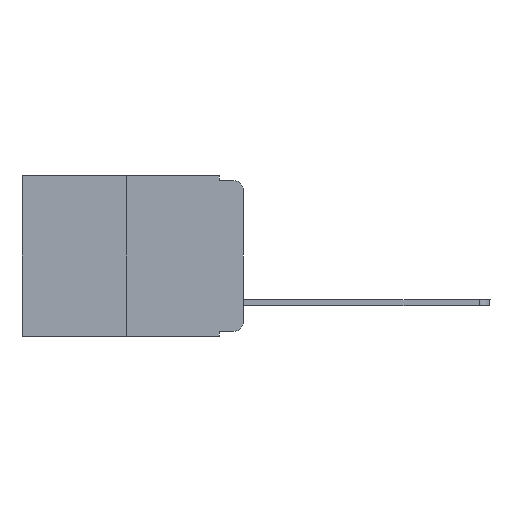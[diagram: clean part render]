
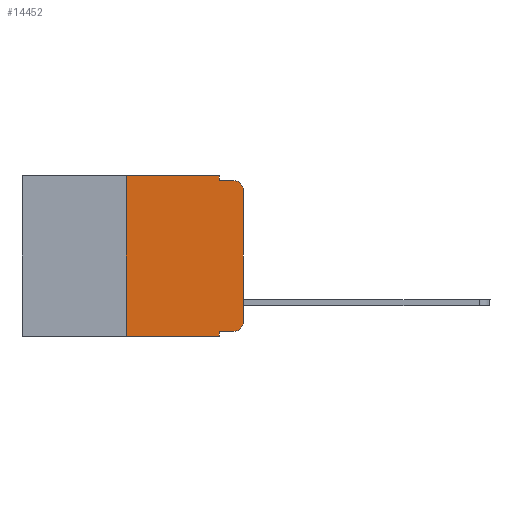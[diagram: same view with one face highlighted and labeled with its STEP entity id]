
A CAD part, left-side view. The second image highlights one B-rep face of the part: STEP entity #14452.
In plain terms, the highlighted planar face has unit normal (-1, 0, 0).
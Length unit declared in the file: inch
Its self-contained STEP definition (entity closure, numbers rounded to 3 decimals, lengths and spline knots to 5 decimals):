
#571 = DIRECTION ( 'NONE',  ( 1., 0., 0. ) ) ;
#807 = VECTOR ( 'NONE', #3811, 39.37008 ) ;
#868 = ORIENTED_EDGE ( 'NONE', *, *, #10553, .T. ) ;
#1630 = EDGE_CURVE ( 'NONE', #2221, #11565, #3370, .T. ) ;
#1830 = CARTESIAN_POINT ( 'NONE',  ( 0., 0.473, 0. ) ) ;
#1958 = VECTOR ( 'NONE', #14750, 39.37008 ) ;
#2143 = PLANE ( 'NONE',  #5240 ) ;
#2221 = VERTEX_POINT ( 'NONE', #19206 ) ;
#2277 = CARTESIAN_POINT ( 'NONE',  ( 0., 0.051, -0.01 ) ) ;
#2434 = DIRECTION ( 'NONE',  ( 0., 0., -1. ) ) ;
#2792 = CARTESIAN_POINT ( 'NONE',  ( 0., 0.051, 0. ) ) ;
#2805 = VECTOR ( 'NONE', #14212, 39.37008 ) ;
#3166 = ORIENTED_EDGE ( 'NONE', *, *, #14502, .T. ) ;
#3370 = LINE ( 'NONE', #14201, #13735 ) ;
#3387 = VECTOR ( 'NONE', #5012, 39.37008 ) ;
#3401 = ORIENTED_EDGE ( 'NONE', *, *, #6089, .T. ) ;
#3436 = VERTEX_POINT ( 'NONE', #17868 ) ;
#3811 = DIRECTION ( 'NONE',  ( 0., -1., 0. ) ) ;
#4032 = LINE ( 'NONE', #1830, #6422 ) ;
#4248 = VERTEX_POINT ( 'NONE', #9648 ) ;
#4620 = VERTEX_POINT ( 'NONE', #11675 ) ;
#4921 = DIRECTION ( 'NONE',  ( 0., 0., 1. ) ) ;
#4950 = CARTESIAN_POINT ( 'NONE',  ( 0., 0.051, -0.343 ) ) ;
#5012 = DIRECTION ( 'NONE',  ( 0., -1., 0. ) ) ;
#5240 = AXIS2_PLACEMENT_3D ( 'NONE', #8316, #571, #12733 ) ;
#5625 = CARTESIAN_POINT ( 'NONE',  ( 0., 0., -0.03 ) ) ;
#6017 = LINE ( 'NONE', #12863, #3387 ) ;
#6089 = EDGE_CURVE ( 'NONE', #4248, #16490, #9199, .T. ) ;
#6422 = VECTOR ( 'NONE', #15561, 39.37008 ) ;
#6891 = ORIENTED_EDGE ( 'NONE', *, *, #16332, .T. ) ;
#8015 = CARTESIAN_POINT ( 'NONE',  ( 0., 0., 0. ) ) ;
#8316 = CARTESIAN_POINT ( 'NONE',  ( 0., 0.473, 0. ) ) ;
#8331 = LINE ( 'NONE', #19037, #2805 ) ;
#8610 = DIRECTION ( 'NONE',  ( -1., 0., 0. ) ) ;
#9040 = CARTESIAN_POINT ( 'NONE',  ( 0., 0.02, -0.01 ) ) ;
#9199 = LINE ( 'NONE', #8015, #15433 ) ;
#9222 = VERTEX_POINT ( 'NONE', #9040 ) ;
#9281 = ORIENTED_EDGE ( 'NONE', *, *, #16196, .F. ) ;
#9462 = ORIENTED_EDGE ( 'NONE', *, *, #19541, .F. ) ;
#9648 = CARTESIAN_POINT ( 'NONE',  ( 0., 0., -0.313 ) ) ;
#9707 = EDGE_CURVE ( 'NONE', #16307, #17786, #10130, .T. ) ;
#9800 = CARTESIAN_POINT ( 'NONE',  ( 0., 0.051, 0. ) ) ;
#9999 = CARTESIAN_POINT ( 'NONE',  ( 0., 0.051, -0.333 ) ) ;
#10130 = LINE ( 'NONE', #2792, #1958 ) ;
#10535 = ORIENTED_EDGE ( 'NONE', *, *, #11070, .T. ) ;
#10553 = EDGE_CURVE ( 'NONE', #16490, #9222, #12452, .T. ) ;
#11070 = EDGE_CURVE ( 'NONE', #4620, #4248, #13889, .T. ) ;
#11306 = FACE_OUTER_BOUND ( 'NONE', #15638, .T. ) ;
#11326 = ORIENTED_EDGE ( 'NONE', *, *, #9707, .F. ) ;
#11565 = VERTEX_POINT ( 'NONE', #14657 ) ;
#11675 = CARTESIAN_POINT ( 'NONE',  ( 0., 0.02, -0.333 ) ) ;
#11723 = CARTESIAN_POINT ( 'NONE',  ( 0., 0.02, -0.03 ) ) ;
#11850 = DIRECTION ( 'NONE',  ( 0., 0., -1. ) ) ;
#12158 = VERTEX_POINT ( 'NONE', #4950 ) ;
#12452 = CIRCLE ( 'NONE', #16785, 0.02 ) ;
#12646 = LINE ( 'NONE', #9999, #14107 ) ;
#12733 = DIRECTION ( 'NONE',  ( 0., 0., -1. ) ) ;
#12863 = CARTESIAN_POINT ( 'NONE',  ( 0., 0.473, -0.343 ) ) ;
#13256 = LINE ( 'NONE', #2277, #807 ) ;
#13735 = VECTOR ( 'NONE', #17268, 39.37008 ) ;
#13889 = CIRCLE ( 'NONE', #19102, 0.02 ) ;
#14107 = VECTOR ( 'NONE', #17711, 39.37008 ) ;
#14201 = CARTESIAN_POINT ( 'NONE',  ( 0., 0.25, 0. ) ) ;
#14212 = DIRECTION ( 'NONE',  ( 0., 0., -1. ) ) ;
#14452 = ADVANCED_FACE ( 'NONE', ( #11306 ), #2143, .F. ) ;
#14502 = EDGE_CURVE ( 'NONE', #2221, #12158, #6017, .T. ) ;
#14657 = CARTESIAN_POINT ( 'NONE',  ( 0., 0.25, 0. ) ) ;
#14694 = ORIENTED_EDGE ( 'NONE', *, *, #16823, .F. ) ;
#14750 = DIRECTION ( 'NONE',  ( 0., 0., -1. ) ) ;
#15433 = VECTOR ( 'NONE', #4921, 39.37008 ) ;
#15561 = DIRECTION ( 'NONE',  ( 0., -1., 0. ) ) ;
#15638 = EDGE_LOOP ( 'NONE', ( #3401, #868, #9462, #11326, #9281, #19136, #3166, #14694, #6891, #10535 ) ) ;
#16196 = EDGE_CURVE ( 'NONE', #11565, #16307, #4032, .T. ) ;
#16307 = VERTEX_POINT ( 'NONE', #9800 ) ;
#16332 = EDGE_CURVE ( 'NONE', #3436, #4620, #12646, .T. ) ;
#16434 = DIRECTION ( 'NONE',  ( -1., 0., 0. ) ) ;
#16490 = VERTEX_POINT ( 'NONE', #5625 ) ;
#16785 = AXIS2_PLACEMENT_3D ( 'NONE', #11723, #16434, #11850 ) ;
#16823 = EDGE_CURVE ( 'NONE', #3436, #12158, #8331, .T. ) ;
#17268 = DIRECTION ( 'NONE',  ( 0., 0., 1. ) ) ;
#17711 = DIRECTION ( 'NONE',  ( 0., -1., 0. ) ) ;
#17786 = VERTEX_POINT ( 'NONE', #18061 ) ;
#17812 = CARTESIAN_POINT ( 'NONE',  ( 0., 0.02, -0.313 ) ) ;
#17868 = CARTESIAN_POINT ( 'NONE',  ( 0., 0.051, -0.333 ) ) ;
#18061 = CARTESIAN_POINT ( 'NONE',  ( 0., 0.051, -0.01 ) ) ;
#19037 = CARTESIAN_POINT ( 'NONE',  ( 0., 0.051, 0. ) ) ;
#19102 = AXIS2_PLACEMENT_3D ( 'NONE', #17812, #8610, #2434 ) ;
#19136 = ORIENTED_EDGE ( 'NONE', *, *, #1630, .F. ) ;
#19206 = CARTESIAN_POINT ( 'NONE',  ( 0., 0.25, -0.343 ) ) ;
#19541 = EDGE_CURVE ( 'NONE', #17786, #9222, #13256, .T. ) ;
